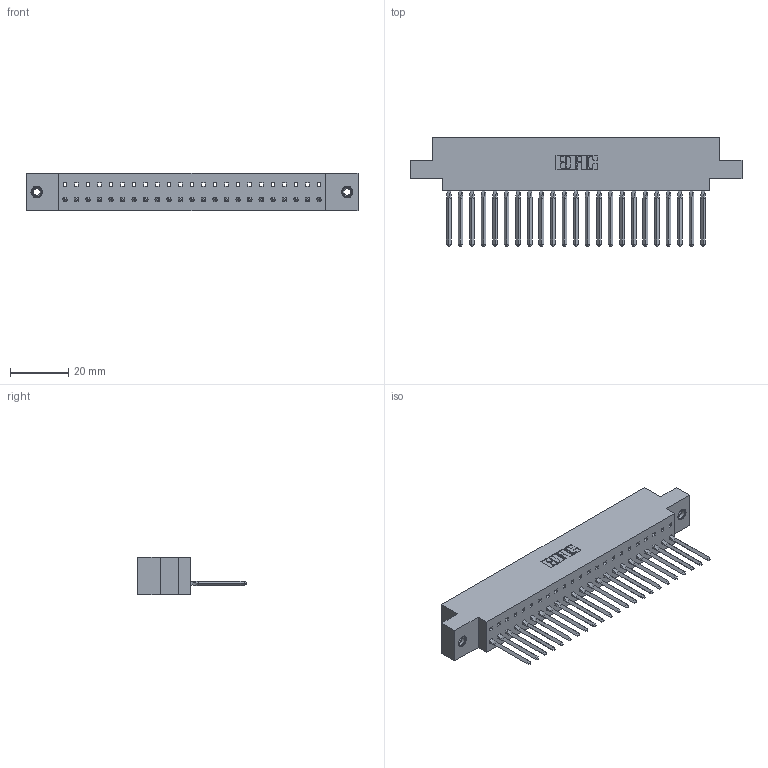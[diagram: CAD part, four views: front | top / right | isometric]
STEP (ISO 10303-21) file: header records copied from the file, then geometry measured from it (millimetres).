
FILE_DESCRIPTION (( 'STEP AP203' ), '1' );
FILE_NAME ('317-023-542-608.STEP', '2020-02-27T17:42:39', ( '' ), ( '' ), 'SwSTEP 2.0', 'SolidWorks 2016', '' );
FILE_SCHEMA (( 'CONFIG_CONTROL_DESIGN' ));
Length unit declared in the file: inch
Products named in the file (4): 317-023-542-608; 317-290-003_542; 317 Part_.156 Dia - TI; 345-250-001_345-250-003-102
Assembly tree (26 placements, depth 2):
  317-023-542-608
    317 Part_.156 Dia - TI
    317-290-003_542  x23
    345-250-001_345-250-003-102  x2
Bounding box: 113.84 x 37.34 x 12.7 mm (x, y, z)
Volume: 17073.9 mm3; surface area: 20425.7 mm2
Topology: 26 solids, 26 shells, 1887 faces, 5402 edges, 3486 vertices
Faces by surface type: plane 1562, cylinder 217, bspline 92, cone 12, torus 4
Entity records: 35364 total; most frequent: CARTESIAN_POINT 6493, ORIENTED_EDGE 6172, DIRECTION 5218, EDGE_CURVE 3086, LINE 2896, VECTOR 2896, VERTEX_POINT 2048, AXIS2_PLACEMENT_3D 1161
